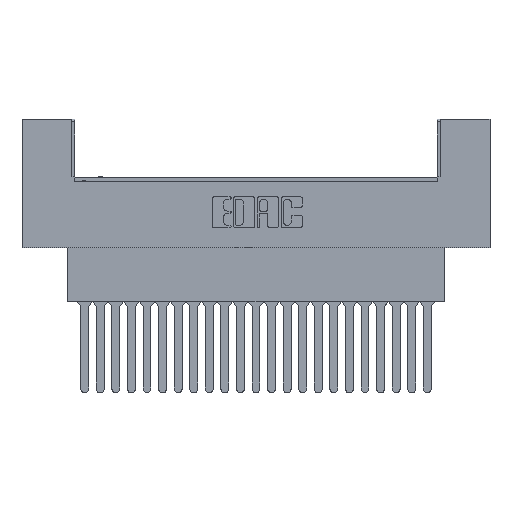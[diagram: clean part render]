
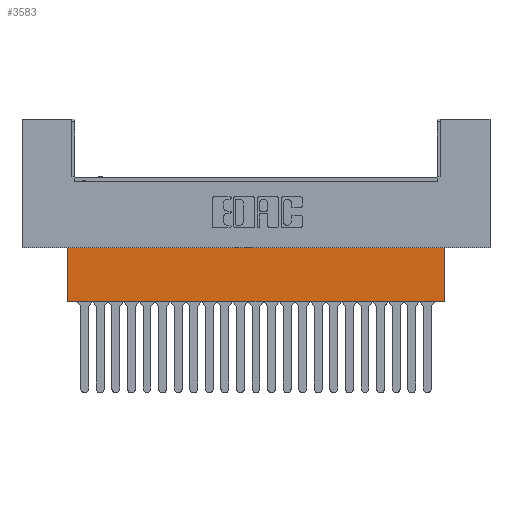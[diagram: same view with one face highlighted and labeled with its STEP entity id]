
A CAD part, top view. The second image highlights one B-rep face of the part: STEP entity #3583.
In plain terms, the highlighted planar face has unit normal (0, 0, 1).
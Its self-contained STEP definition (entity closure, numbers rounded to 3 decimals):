
#601 = VERTEX_POINT ( 'NONE', #9540 ) ;
#1512 = LINE ( 'NONE', #29224, #23849 ) ;
#1659 = EDGE_CURVE ( 'NONE', #23658, #22988, #5104, .T. ) ;
#1705 = EDGE_CURVE ( 'NONE', #601, #23658, #1512, .T. ) ;
#2482 = CARTESIAN_POINT ( 'NONE',  ( 7.468, -8.814, -3.962 ) ) ;
#3360 = DIRECTION ( 'NONE',  ( 0., 0., -1. ) ) ;
#3583 = ADVANCED_FACE ( 'NONE', ( #15259 ), #16910, .F. ) ;
#3809 = CARTESIAN_POINT ( 'NONE',  ( 7.468, 0., -3.962 ) ) ;
#4588 = VECTOR ( 'NONE', #27905, 1000. ) ;
#5104 = LINE ( 'NONE', #17101, #22810 ) ;
#6136 = VERTEX_POINT ( 'NONE', #3809 ) ;
#6668 = ORIENTED_EDGE ( 'NONE', *, *, #24421, .F. ) ;
#7512 = DIRECTION ( 'NONE',  ( 0., 1., 0. ) ) ;
#8216 = EDGE_LOOP ( 'NONE', ( #24832, #19077, #12051, #6668 ) ) ;
#9412 = EDGE_CURVE ( 'NONE', #601, #6136, #23367, .T. ) ;
#9540 = CARTESIAN_POINT ( 'NONE',  ( 68.885, 0., -3.962 ) ) ;
#12051 = ORIENTED_EDGE ( 'NONE', *, *, #9412, .T. ) ;
#13415 = AXIS2_PLACEMENT_3D ( 'NONE', #19127, #3360, #7512 ) ;
#13448 = LINE ( 'NONE', #16103, #29631 ) ;
#15259 = FACE_OUTER_BOUND ( 'NONE', #8216, .T. ) ;
#16103 = CARTESIAN_POINT ( 'NONE',  ( 7.468, -8.814, -3.962 ) ) ;
#16910 = PLANE ( 'NONE',  #13415 ) ;
#17101 = CARTESIAN_POINT ( 'NONE',  ( 76.352, -8.814, -3.962 ) ) ;
#18503 = DIRECTION ( 'NONE',  ( 0., 1., 0. ) ) ;
#19077 = ORIENTED_EDGE ( 'NONE', *, *, #1705, .F. ) ;
#19127 = CARTESIAN_POINT ( 'NONE',  ( 76.352, 0., -3.962 ) ) ;
#19517 = DIRECTION ( 'NONE',  ( -1., 0., 0. ) ) ;
#20565 = CARTESIAN_POINT ( 'NONE',  ( 68.885, -8.814, -3.962 ) ) ;
#22810 = VECTOR ( 'NONE', #19517, 1000. ) ;
#22988 = VERTEX_POINT ( 'NONE', #2482 ) ;
#23367 = LINE ( 'NONE', #25879, #4588 ) ;
#23658 = VERTEX_POINT ( 'NONE', #20565 ) ;
#23849 = VECTOR ( 'NONE', #24811, 1000. ) ;
#24421 = EDGE_CURVE ( 'NONE', #22988, #6136, #13448, .T. ) ;
#24811 = DIRECTION ( 'NONE',  ( 0., -1., 0. ) ) ;
#24832 = ORIENTED_EDGE ( 'NONE', *, *, #1659, .F. ) ;
#25879 = CARTESIAN_POINT ( 'NONE',  ( 76.352, 0., -3.962 ) ) ;
#27905 = DIRECTION ( 'NONE',  ( -1., 0., 0. ) ) ;
#29224 = CARTESIAN_POINT ( 'NONE',  ( 68.885, -8.814, -3.962 ) ) ;
#29631 = VECTOR ( 'NONE', #18503, 1000. ) ;
